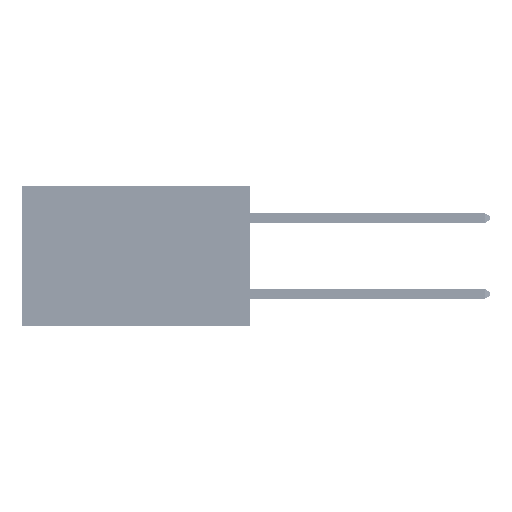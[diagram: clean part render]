
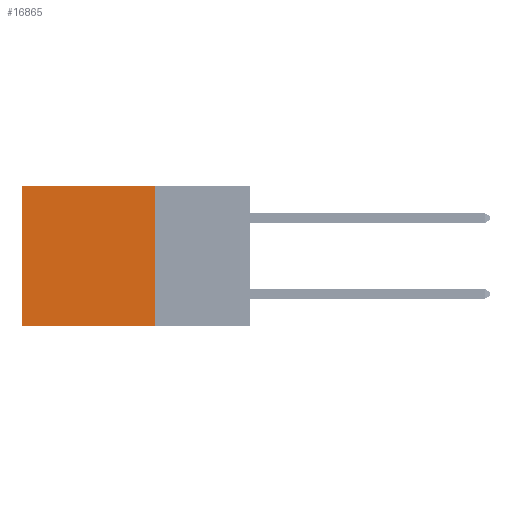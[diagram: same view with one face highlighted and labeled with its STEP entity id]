
A CAD part, left-side view. The second image highlights one B-rep face of the part: STEP entity #16865.
In plain terms, the highlighted planar face has unit normal (-1, 0, 0).
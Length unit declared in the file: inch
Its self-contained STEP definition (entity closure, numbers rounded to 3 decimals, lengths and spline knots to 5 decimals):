
#696 = DIRECTION ( 'NONE',  ( 0., 0., -1. ) ) ;
#3589 = DIRECTION ( 'NONE',  ( 0., 1., 0. ) ) ;
#7944 = ORIENTED_EDGE ( 'NONE', *, *, #42568, .F. ) ;
#9954 = EDGE_CURVE ( 'NONE', #34458, #26007, #20687, .T. ) ;
#10650 = PLANE ( 'NONE',  #26617 ) ;
#11157 = DIRECTION ( 'NONE',  ( 0., 0., -1. ) ) ;
#12283 = VECTOR ( 'NONE', #36794, 39.37008 ) ;
#12383 = EDGE_CURVE ( 'NONE', #26007, #47247, #32545, .T. ) ;
#13610 = ORIENTED_EDGE ( 'NONE', *, *, #9954, .T. ) ;
#14528 = CARTESIAN_POINT ( 'NONE',  ( 0.2875, 0.25, 0. ) ) ;
#16865 = ADVANCED_FACE ( 'NONE', ( #40860 ), #10650, .F. ) ;
#18532 = DIRECTION ( 'NONE',  ( 1., 0., 0. ) ) ;
#20671 = VERTEX_POINT ( 'NONE', #39096 ) ;
#20687 = LINE ( 'NONE', #47873, #12283 ) ;
#22620 = CARTESIAN_POINT ( 'NONE',  ( 0.2875, 0.25, 0. ) ) ;
#24862 = CARTESIAN_POINT ( 'NONE',  ( 0.2875, 0.6, -0.37 ) ) ;
#24999 = ORIENTED_EDGE ( 'NONE', *, *, #47684, .F. ) ;
#25122 = CARTESIAN_POINT ( 'NONE',  ( 0.2875, 0.6, 0. ) ) ;
#25532 = LINE ( 'NONE', #49584, #29724 ) ;
#26007 = VERTEX_POINT ( 'NONE', #48585 ) ;
#26617 = AXIS2_PLACEMENT_3D ( 'NONE', #22620, #18532, #11157 ) ;
#29724 = VECTOR ( 'NONE', #3589, 39.37008 ) ;
#32528 = DIRECTION ( 'NONE',  ( 0., 0., -1. ) ) ;
#32545 = LINE ( 'NONE', #25122, #45204 ) ;
#34458 = VERTEX_POINT ( 'NONE', #14528 ) ;
#36794 = DIRECTION ( 'NONE',  ( 0., 1., 0. ) ) ;
#37685 = LINE ( 'NONE', #47005, #38891 ) ;
#38891 = VECTOR ( 'NONE', #696, 39.37008 ) ;
#39096 = CARTESIAN_POINT ( 'NONE',  ( 0.2875, 0.25, -0.37 ) ) ;
#40065 = ORIENTED_EDGE ( 'NONE', *, *, #12383, .T. ) ;
#40860 = FACE_OUTER_BOUND ( 'NONE', #47130, .T. ) ;
#42568 = EDGE_CURVE ( 'NONE', #20671, #47247, #25532, .T. ) ;
#45204 = VECTOR ( 'NONE', #32528, 39.37008 ) ;
#47005 = CARTESIAN_POINT ( 'NONE',  ( 0.2875, 0.25, 0. ) ) ;
#47130 = EDGE_LOOP ( 'NONE', ( #40065, #7944, #24999, #13610 ) ) ;
#47247 = VERTEX_POINT ( 'NONE', #24862 ) ;
#47684 = EDGE_CURVE ( 'NONE', #34458, #20671, #37685, .T. ) ;
#47873 = CARTESIAN_POINT ( 'NONE',  ( 0.2875, 0.25, 0. ) ) ;
#48585 = CARTESIAN_POINT ( 'NONE',  ( 0.2875, 0.6, 0. ) ) ;
#49584 = CARTESIAN_POINT ( 'NONE',  ( 0.2875, 0.25, -0.37 ) ) ;
